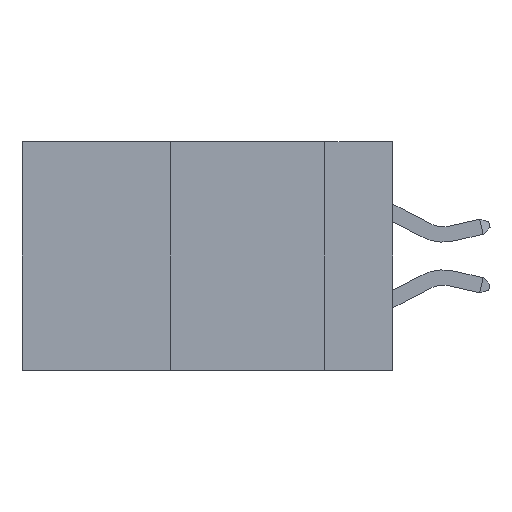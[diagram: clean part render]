
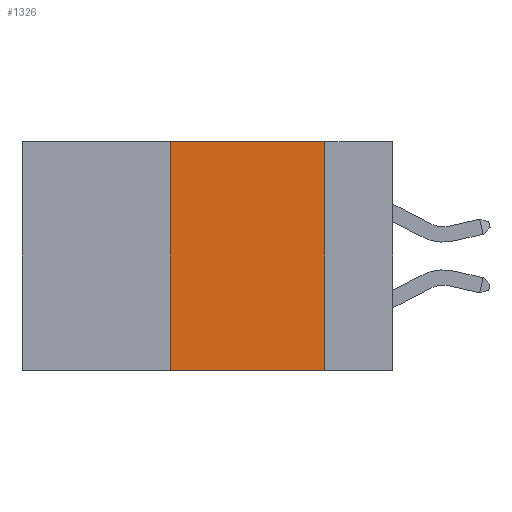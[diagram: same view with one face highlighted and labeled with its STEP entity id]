
A CAD part, left-side view. The second image highlights one B-rep face of the part: STEP entity #1326.
In plain terms, the highlighted planar face has unit normal (-1, 0, 0).
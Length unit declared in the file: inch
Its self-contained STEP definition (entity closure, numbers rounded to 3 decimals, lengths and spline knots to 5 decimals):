
#517 = FACE_OUTER_BOUND ( 'NONE', #13995, .T. ) ;
#697 = LINE ( 'NONE', #8485, #18990 ) ;
#1326 = ADVANCED_FACE ( 'NONE', ( #517 ), #6533, .F. ) ;
#1552 = EDGE_CURVE ( 'NONE', #7610, #15912, #6112, .T. ) ;
#2132 = ORIENTED_EDGE ( 'NONE', *, *, #4012, .T. ) ;
#3286 = CARTESIAN_POINT ( 'NONE',  ( 0., 0.36, 0. ) ) ;
#3927 = DIRECTION ( 'NONE',  ( 0., -1., 0. ) ) ;
#3959 = ORIENTED_EDGE ( 'NONE', *, *, #15429, .F. ) ;
#4012 = EDGE_CURVE ( 'NONE', #4736, #11248, #17493, .T. ) ;
#4736 = VERTEX_POINT ( 'NONE', #11059 ) ;
#6112 = LINE ( 'NONE', #7294, #16938 ) ;
#6533 = PLANE ( 'NONE',  #18724 ) ;
#6883 = VECTOR ( 'NONE', #9740, 39.37008 ) ;
#7111 = DIRECTION ( 'NONE',  ( 0., 0., -1. ) ) ;
#7185 = EDGE_CURVE ( 'NONE', #15912, #11248, #11215, .T. ) ;
#7257 = CARTESIAN_POINT ( 'NONE',  ( 0., 0.6, -0.37 ) ) ;
#7294 = CARTESIAN_POINT ( 'NONE',  ( 0., 0.6, 0. ) ) ;
#7610 = VERTEX_POINT ( 'NONE', #3286 ) ;
#8485 = CARTESIAN_POINT ( 'NONE',  ( 0., 0.36, 0. ) ) ;
#9740 = DIRECTION ( 'NONE',  ( 0., 0., -1. ) ) ;
#9949 = ORIENTED_EDGE ( 'NONE', *, *, #7185, .F. ) ;
#11059 = CARTESIAN_POINT ( 'NONE',  ( 0., 0.36, -0.37 ) ) ;
#11215 = LINE ( 'NONE', #17212, #6883 ) ;
#11248 = VERTEX_POINT ( 'NONE', #13093 ) ;
#11591 = ORIENTED_EDGE ( 'NONE', *, *, #1552, .F. ) ;
#11916 = DIRECTION ( 'NONE',  ( 0., -1., 0. ) ) ;
#12524 = CARTESIAN_POINT ( 'NONE',  ( 0., 0.6, 0. ) ) ;
#13093 = CARTESIAN_POINT ( 'NONE',  ( 0., 0.11, -0.37 ) ) ;
#13995 = EDGE_LOOP ( 'NONE', ( #9949, #11591, #3959, #2132 ) ) ;
#14959 = VECTOR ( 'NONE', #3927, 39.37008 ) ;
#15429 = EDGE_CURVE ( 'NONE', #4736, #7610, #697, .T. ) ;
#15912 = VERTEX_POINT ( 'NONE', #19054 ) ;
#15964 = DIRECTION ( 'NONE',  ( 0., 0., 1. ) ) ;
#16938 = VECTOR ( 'NONE', #11916, 39.37008 ) ;
#17212 = CARTESIAN_POINT ( 'NONE',  ( 0., 0.11, 0. ) ) ;
#17493 = LINE ( 'NONE', #7257, #14959 ) ;
#18724 = AXIS2_PLACEMENT_3D ( 'NONE', #12524, #18908, #7111 ) ;
#18908 = DIRECTION ( 'NONE',  ( 1., 0., 0. ) ) ;
#18990 = VECTOR ( 'NONE', #15964, 39.37008 ) ;
#19054 = CARTESIAN_POINT ( 'NONE',  ( 0., 0.11, 0. ) ) ;
